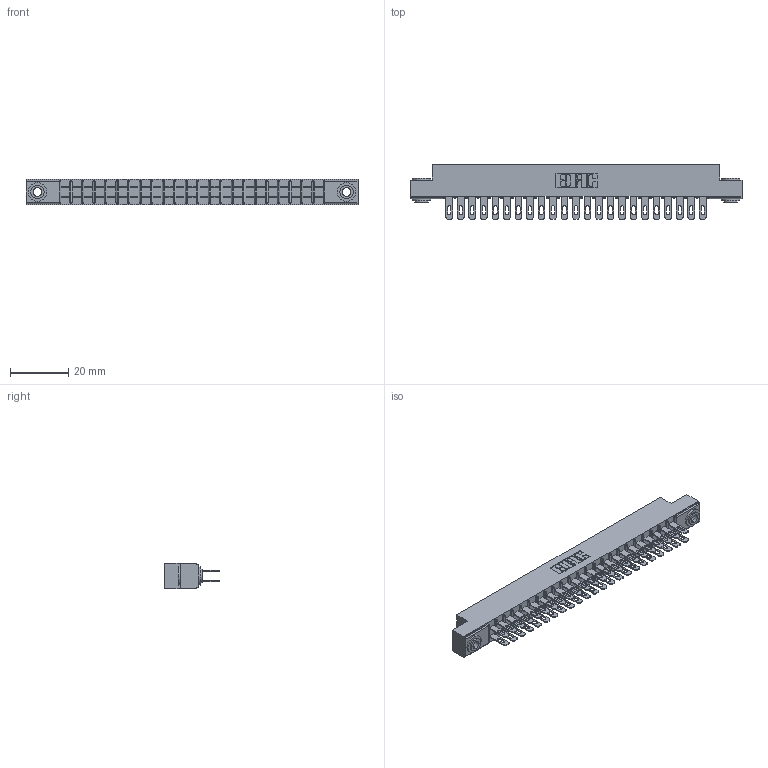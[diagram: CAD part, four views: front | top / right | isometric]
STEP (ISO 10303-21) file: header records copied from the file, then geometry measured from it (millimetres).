
FILE_DESCRIPTION (( 'STEP AP203' ), '1' );
FILE_NAME ('355-046-500-203.STEP', '2019-09-11T14:29:54', ( '' ), ( '' ), 'SwSTEP 2.0', 'SolidWorks 2016', '' );
FILE_SCHEMA (( 'CONFIG_CONTROL_DESIGN' ));
Length unit declared in the file: inch
Products named in the file (4): 345-250-002_345-250-002-102; 305 Part_.156 Dia; 355-046-500-203; 305-290-001_500
Assembly tree (49 placements, depth 2):
  355-046-500-203
    305 Part_.156 Dia
    305-290-001_500  x46
    345-250-002_345-250-002-102  x2
Bounding box: 114.15 x 18.85 x 8.71 mm (x, y, z)
Volume: 7296.8 mm3; surface area: 14906.9 mm2
Topology: 49 solids, 49 shells, 2468 faces, 7029 edges, 4558 vertices
Faces by surface type: plane 1380, cylinder 988, sphere 92, cone 8
Entity records: 28303 total; most frequent: CARTESIAN_POINT 4664, ORIENTED_EDGE 4618, DIRECTION 4545, EDGE_CURVE 2309, VECTOR 1835, LINE 1835, VERTEX_POINT 1474, AXIS2_PLACEMENT_3D 1355
